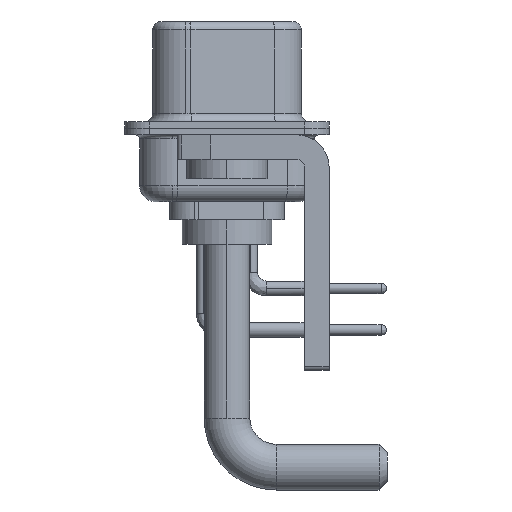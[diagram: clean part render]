
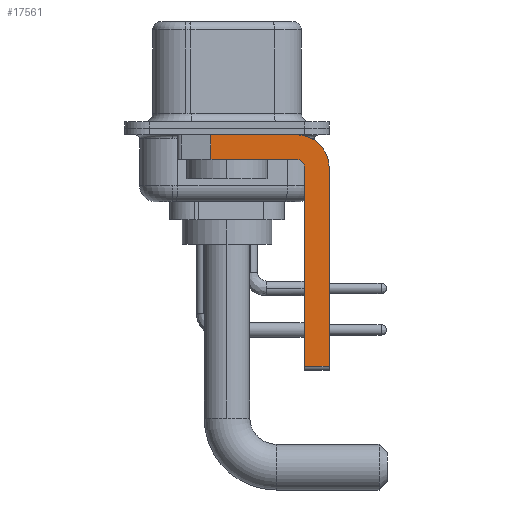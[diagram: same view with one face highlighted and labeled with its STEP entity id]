
A CAD part, left-side view. The second image highlights one B-rep face of the part: STEP entity #17561.
In plain terms, the highlighted planar face has unit normal (-1, 0, 0).
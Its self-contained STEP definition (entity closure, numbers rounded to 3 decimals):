
#677 = DIRECTION ( 'NONE',  ( 0., 0., 1. ) ) ;
#1138 = CARTESIAN_POINT ( 'NONE',  ( -2.9, -6.25, -14.55 ) ) ;
#1236 = DIRECTION ( 'NONE',  ( 0., 0., 1. ) ) ;
#1461 = VECTOR ( 'NONE', #2000, 1000. ) ;
#1954 = DIRECTION ( 'NONE',  ( 1., 0., 0. ) ) ;
#2000 = DIRECTION ( 'NONE',  ( 0., 0., -1. ) ) ;
#2492 = CARTESIAN_POINT ( 'NONE',  ( -2.9, 3., -0.4 ) ) ;
#2561 = AXIS2_PLACEMENT_3D ( 'NONE', #23354, #8926, #4720 ) ;
#3032 = VECTOR ( 'NONE', #15396, 1000. ) ;
#3973 = LINE ( 'NONE', #6494, #1461 ) ;
#4514 = ORIENTED_EDGE ( 'NONE', *, *, #6758, .F. ) ;
#4621 = ORIENTED_EDGE ( 'NONE', *, *, #23399, .T. ) ;
#4720 = DIRECTION ( 'NONE',  ( 0., 0., -1. ) ) ;
#4875 = CARTESIAN_POINT ( 'NONE',  ( -2.9, -4.75, -2.4 ) ) ;
#5095 = EDGE_LOOP ( 'NONE', ( #22331, #21923, #15345, #12897, #4514, #4621, #5185, #6773 ) ) ;
#5185 = ORIENTED_EDGE ( 'NONE', *, *, #18423, .F. ) ;
#6034 = CIRCLE ( 'NONE', #18579, 0.5 ) ;
#6161 = CARTESIAN_POINT ( 'NONE',  ( -2.9, -4.25, -2.4 ) ) ;
#6494 = CARTESIAN_POINT ( 'NONE',  ( -2.9, 0.978, -1.9 ) ) ;
#6758 = EDGE_CURVE ( 'NONE', #17786, #25050, #15949, .T. ) ;
#6773 = ORIENTED_EDGE ( 'NONE', *, *, #8224, .F. ) ;
#6903 = DIRECTION ( 'NONE',  ( 0., -1., 0. ) ) ;
#7115 = CARTESIAN_POINT ( 'NONE',  ( -2.9, -4.25, -1.9 ) ) ;
#8224 = EDGE_CURVE ( 'NONE', #25677, #21548, #23162, .T. ) ;
#8683 = EDGE_CURVE ( 'NONE', #10967, #25677, #25888, .T. ) ;
#8820 = EDGE_CURVE ( 'NONE', #27462, #21882, #19175, .T. ) ;
#8926 = DIRECTION ( 'NONE',  ( 1., 0., 0. ) ) ;
#9135 = CARTESIAN_POINT ( 'NONE',  ( -2.9, -4.25, -0.4 ) ) ;
#9180 = CARTESIAN_POINT ( 'NONE',  ( -2.9, 0.978, -1.9 ) ) ;
#10086 = VECTOR ( 'NONE', #24590, 1000. ) ;
#10954 = AXIS2_PLACEMENT_3D ( 'NONE', #6161, #1954, #16536 ) ;
#10967 = VERTEX_POINT ( 'NONE', #19783 ) ;
#11181 = VECTOR ( 'NONE', #677, 1000. ) ;
#11535 = LINE ( 'NONE', #26091, #23799 ) ;
#11628 = CARTESIAN_POINT ( 'NONE',  ( -2.9, -4.75, -14.8 ) ) ;
#11910 = DIRECTION ( 'NONE',  ( -1., 0., 0. ) ) ;
#12876 = DIRECTION ( 'NONE',  ( 0., 1., 0. ) ) ;
#12897 = ORIENTED_EDGE ( 'NONE', *, *, #18043, .F. ) ;
#13964 = CARTESIAN_POINT ( 'NONE',  ( -2.9, -6.25, -2.4 ) ) ;
#15345 = ORIENTED_EDGE ( 'NONE', *, *, #8820, .F. ) ;
#15396 = DIRECTION ( 'NONE',  ( 0., -1., 0. ) ) ;
#15949 = LINE ( 'NONE', #11628, #11181 ) ;
#16047 = LINE ( 'NONE', #13964, #10086 ) ;
#16048 = CARTESIAN_POINT ( 'NONE',  ( -2.9, -6.25, -2.4 ) ) ;
#16536 = DIRECTION ( 'NONE',  ( 0., 0., -1. ) ) ;
#17561 = ADVANCED_FACE ( 'NONE', ( #27479 ), #20880, .F. ) ;
#17786 = VERTEX_POINT ( 'NONE', #20164 ) ;
#18043 = EDGE_CURVE ( 'NONE', #25050, #27462, #6034, .T. ) ;
#18339 = CARTESIAN_POINT ( 'NONE',  ( -2.9, -4.25, -2.4 ) ) ;
#18423 = EDGE_CURVE ( 'NONE', #21548, #25765, #16047, .T. ) ;
#18579 = AXIS2_PLACEMENT_3D ( 'NONE', #18339, #11910, #1236 ) ;
#19175 = LINE ( 'NONE', #27740, #24514 ) ;
#19783 = CARTESIAN_POINT ( 'NONE',  ( -2.9, 0.978, -0.4 ) ) ;
#20164 = CARTESIAN_POINT ( 'NONE',  ( -2.9, -4.75, -14.55 ) ) ;
#20880 = PLANE ( 'NONE',  #10954 ) ;
#21548 = VERTEX_POINT ( 'NONE', #16048 ) ;
#21882 = VERTEX_POINT ( 'NONE', #9180 ) ;
#21923 = ORIENTED_EDGE ( 'NONE', *, *, #23212, .T. ) ;
#22331 = ORIENTED_EDGE ( 'NONE', *, *, #8683, .F. ) ;
#23162 = CIRCLE ( 'NONE', #2561, 2. ) ;
#23212 = EDGE_CURVE ( 'NONE', #10967, #21882, #3973, .T. ) ;
#23354 = CARTESIAN_POINT ( 'NONE',  ( -2.9, -4.25, -2.4 ) ) ;
#23399 = EDGE_CURVE ( 'NONE', #17786, #25765, #11535, .T. ) ;
#23799 = VECTOR ( 'NONE', #6903, 1000. ) ;
#24514 = VECTOR ( 'NONE', #12876, 1000. ) ;
#24590 = DIRECTION ( 'NONE',  ( 0., 0., -1. ) ) ;
#25050 = VERTEX_POINT ( 'NONE', #4875 ) ;
#25677 = VERTEX_POINT ( 'NONE', #9135 ) ;
#25765 = VERTEX_POINT ( 'NONE', #1138 ) ;
#25888 = LINE ( 'NONE', #2492, #3032 ) ;
#26091 = CARTESIAN_POINT ( 'NONE',  ( -2.9, -4.25, -14.55 ) ) ;
#27462 = VERTEX_POINT ( 'NONE', #7115 ) ;
#27479 = FACE_OUTER_BOUND ( 'NONE', #5095, .T. ) ;
#27740 = CARTESIAN_POINT ( 'NONE',  ( -2.9, -4.25, -1.9 ) ) ;
